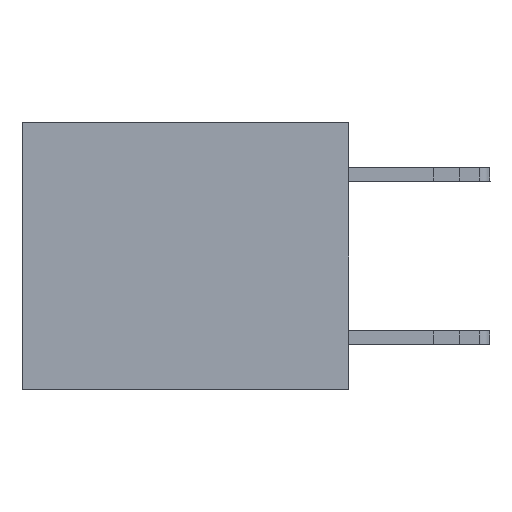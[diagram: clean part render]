
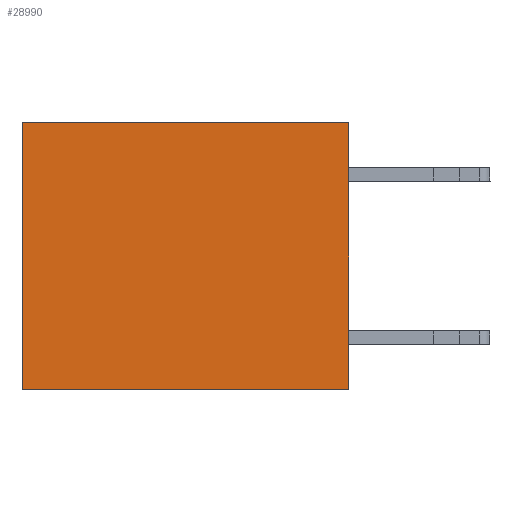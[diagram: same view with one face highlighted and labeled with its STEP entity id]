
A CAD part, left-side view. The second image highlights one B-rep face of the part: STEP entity #28990.
In plain terms, the highlighted planar face has unit normal (-1, 0, 0).
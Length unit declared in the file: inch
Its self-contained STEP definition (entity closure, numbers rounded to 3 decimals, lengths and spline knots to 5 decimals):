
#386 = VECTOR ( 'NONE', #27218, 39.37008 ) ;
#1513 = CARTESIAN_POINT ( 'NONE',  ( 0.3165, 0., -0.49 ) ) ;
#1787 = VECTOR ( 'NONE', #29642, 39.37008 ) ;
#1818 = CARTESIAN_POINT ( 'NONE',  ( 0.3165, 0., 0. ) ) ;
#2033 = CARTESIAN_POINT ( 'NONE',  ( 0.3165, 0., -0.49 ) ) ;
#6967 = VECTOR ( 'NONE', #27438, 39.37008 ) ;
#7208 = CARTESIAN_POINT ( 'NONE',  ( 0.3165, 0., -0.49 ) ) ;
#7798 = FACE_OUTER_BOUND ( 'NONE', #22284, .T. ) ;
#9066 = DIRECTION ( 'NONE',  ( 0., 0., -1. ) ) ;
#9079 = ORIENTED_EDGE ( 'NONE', *, *, #20609, .F. ) ;
#11230 = LINE ( 'NONE', #1513, #30273 ) ;
#11761 = CARTESIAN_POINT ( 'NONE',  ( 0.3165, 0.6, -0.49 ) ) ;
#13529 = AXIS2_PLACEMENT_3D ( 'NONE', #29185, #26429, #9066 ) ;
#13543 = ORIENTED_EDGE ( 'NONE', *, *, #25449, .T. ) ;
#14622 = ORIENTED_EDGE ( 'NONE', *, *, #21176, .T. ) ;
#18994 = PLANE ( 'NONE',  #13529 ) ;
#20609 = EDGE_CURVE ( 'NONE', #20901, #24438, #21545, .T. ) ;
#20795 = LINE ( 'NONE', #11761, #1787 ) ;
#20901 = VERTEX_POINT ( 'NONE', #7208 ) ;
#21176 = EDGE_CURVE ( 'NONE', #21968, #24438, #20795, .T. ) ;
#21545 = LINE ( 'NONE', #2033, #6967 ) ;
#21968 = VERTEX_POINT ( 'NONE', #32403 ) ;
#22284 = EDGE_LOOP ( 'NONE', ( #14622, #9079, #29191, #13543 ) ) ;
#23545 = VERTEX_POINT ( 'NONE', #30428 ) ;
#24309 = DIRECTION ( 'NONE',  ( 0., 0., -1. ) ) ;
#24438 = VERTEX_POINT ( 'NONE', #24488 ) ;
#24488 = CARTESIAN_POINT ( 'NONE',  ( 0.3165, 0.6, -0.49 ) ) ;
#25449 = EDGE_CURVE ( 'NONE', #23545, #21968, #27357, .T. ) ;
#26429 = DIRECTION ( 'NONE',  ( 1., 0., 0. ) ) ;
#27218 = DIRECTION ( 'NONE',  ( 0., 1., 0. ) ) ;
#27357 = LINE ( 'NONE', #1818, #386 ) ;
#27438 = DIRECTION ( 'NONE',  ( 0., 1., 0. ) ) ;
#27455 = EDGE_CURVE ( 'NONE', #23545, #20901, #11230, .T. ) ;
#28990 = ADVANCED_FACE ( 'NONE', ( #7798 ), #18994, .F. ) ;
#29185 = CARTESIAN_POINT ( 'NONE',  ( 0.3165, 0., -0.49 ) ) ;
#29191 = ORIENTED_EDGE ( 'NONE', *, *, #27455, .F. ) ;
#29642 = DIRECTION ( 'NONE',  ( 0., 0., -1. ) ) ;
#30273 = VECTOR ( 'NONE', #24309, 39.37008 ) ;
#30428 = CARTESIAN_POINT ( 'NONE',  ( 0.3165, 0., 0. ) ) ;
#32403 = CARTESIAN_POINT ( 'NONE',  ( 0.3165, 0.6, 0. ) ) ;
